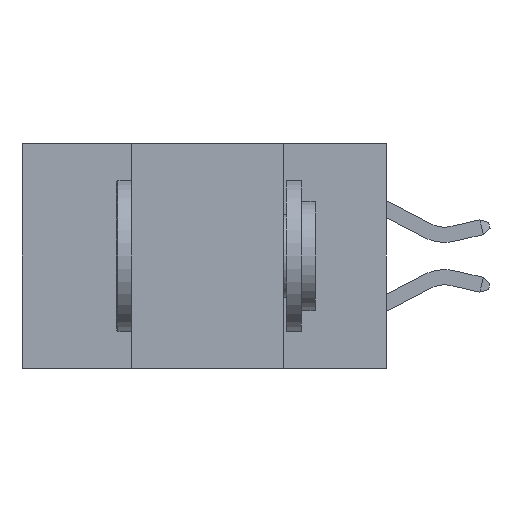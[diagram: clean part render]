
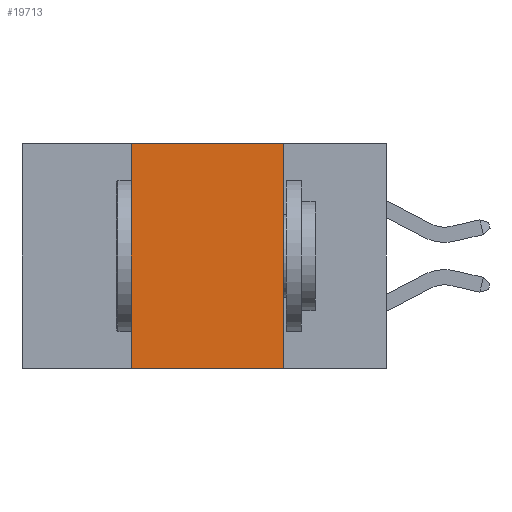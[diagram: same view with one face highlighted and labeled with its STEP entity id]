
A CAD part, left-side view. The second image highlights one B-rep face of the part: STEP entity #19713.
In plain terms, the highlighted planar face has unit normal (-1, 0, 0).
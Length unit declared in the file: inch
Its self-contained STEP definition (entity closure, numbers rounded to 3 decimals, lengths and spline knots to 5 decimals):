
#19 = CARTESIAN_POINT ( 'NONE',  ( 0., 0.42, -0.37 ) ) ;
#1776 = LINE ( 'NONE', #18724, #12017 ) ;
#2011 = EDGE_LOOP ( 'NONE', ( #3129, #5329, #17996, #16168 ) ) ;
#2144 = VERTEX_POINT ( 'NONE', #15032 ) ;
#2400 = VECTOR ( 'NONE', #2906, 39.37008 ) ;
#2876 = DIRECTION ( 'NONE',  ( 0., -1., 0. ) ) ;
#2906 = DIRECTION ( 'NONE',  ( 0., 0., -1. ) ) ;
#3129 = ORIENTED_EDGE ( 'NONE', *, *, #11863, .F. ) ;
#3994 = DIRECTION ( 'NONE',  ( 1., 0., 0. ) ) ;
#4043 = VECTOR ( 'NONE', #10267, 39.37008 ) ;
#4492 = CARTESIAN_POINT ( 'NONE',  ( 0., 0.6, -0.37 ) ) ;
#4753 = CARTESIAN_POINT ( 'NONE',  ( 0., 0.17, -0.37 ) ) ;
#5300 = CARTESIAN_POINT ( 'NONE',  ( 0., 0.6, 0. ) ) ;
#5329 = ORIENTED_EDGE ( 'NONE', *, *, #11208, .F. ) ;
#6712 = VERTEX_POINT ( 'NONE', #9429 ) ;
#7054 = CARTESIAN_POINT ( 'NONE',  ( 0., 0.42, -0.37 ) ) ;
#8295 = DIRECTION ( 'NONE',  ( 0., 0., -1. ) ) ;
#8925 = LINE ( 'NONE', #16663, #2400 ) ;
#9429 = CARTESIAN_POINT ( 'NONE',  ( 0., 0.42, 0. ) ) ;
#10267 = DIRECTION ( 'NONE',  ( 0., 0., 1. ) ) ;
#10556 = EDGE_CURVE ( 'NONE', #18454, #6712, #18387, .T. ) ;
#11208 = EDGE_CURVE ( 'NONE', #6712, #2144, #1776, .T. ) ;
#11863 = EDGE_CURVE ( 'NONE', #2144, #17223, #8925, .T. ) ;
#12017 = VECTOR ( 'NONE', #12723, 39.37008 ) ;
#12723 = DIRECTION ( 'NONE',  ( 0., -1., 0. ) ) ;
#14224 = AXIS2_PLACEMENT_3D ( 'NONE', #5300, #3994, #8295 ) ;
#15032 = CARTESIAN_POINT ( 'NONE',  ( 0., 0.17, 0. ) ) ;
#16024 = PLANE ( 'NONE',  #14224 ) ;
#16168 = ORIENTED_EDGE ( 'NONE', *, *, #16291, .T. ) ;
#16291 = EDGE_CURVE ( 'NONE', #18454, #17223, #16631, .T. ) ;
#16631 = LINE ( 'NONE', #4492, #19528 ) ;
#16663 = CARTESIAN_POINT ( 'NONE',  ( 0., 0.17, -0.37 ) ) ;
#17223 = VERTEX_POINT ( 'NONE', #4753 ) ;
#17996 = ORIENTED_EDGE ( 'NONE', *, *, #10556, .F. ) ;
#18387 = LINE ( 'NONE', #19, #4043 ) ;
#18454 = VERTEX_POINT ( 'NONE', #7054 ) ;
#18724 = CARTESIAN_POINT ( 'NONE',  ( 0., 0.6, 0. ) ) ;
#19458 = FACE_OUTER_BOUND ( 'NONE', #2011, .T. ) ;
#19528 = VECTOR ( 'NONE', #2876, 39.37008 ) ;
#19713 = ADVANCED_FACE ( 'NONE', ( #19458 ), #16024, .F. ) ;
